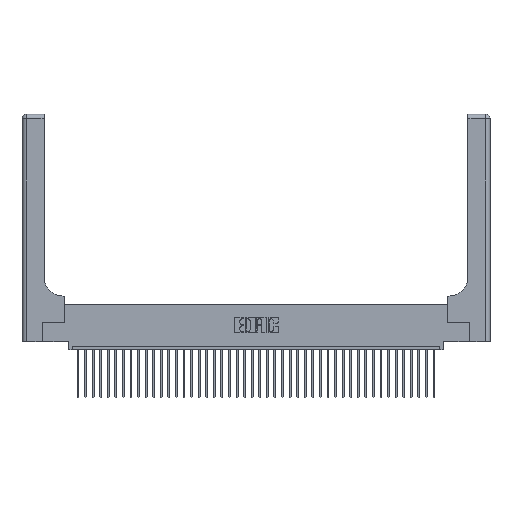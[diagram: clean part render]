
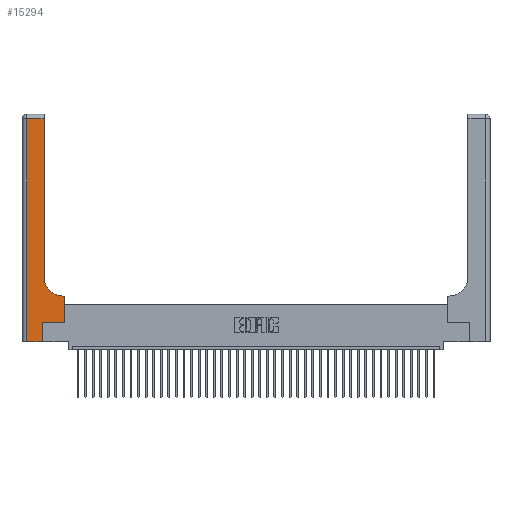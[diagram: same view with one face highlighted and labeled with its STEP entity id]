
A CAD part, top view. The second image highlights one B-rep face of the part: STEP entity #15294.
In plain terms, the highlighted planar face has unit normal (0, 0, 1).
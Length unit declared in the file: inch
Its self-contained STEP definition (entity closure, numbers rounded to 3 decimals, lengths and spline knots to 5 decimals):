
#900 = ORIENTED_EDGE ( 'NONE', *, *, #3843, .T. ) ;
#986 = DIRECTION ( 'NONE',  ( -1., 0., 0. ) ) ;
#2091 = CARTESIAN_POINT ( 'NONE',  ( 0.5585, 0.6, 0.37 ) ) ;
#2290 = EDGE_CURVE ( 'NONE', #22483, #12610, #5214, .T. ) ;
#2780 = CARTESIAN_POINT ( 'NONE',  ( 0.269, 0.25, 0.37 ) ) ;
#3843 = EDGE_CURVE ( 'NONE', #22771, #7628, #37944, .T. ) ;
#5178 = DIRECTION ( 'NONE',  ( -1., 0., 0. ) ) ;
#5214 = LINE ( 'NONE', #17101, #18475 ) ;
#5258 = CARTESIAN_POINT ( 'NONE',  ( 0.269, 0.25, 0.37 ) ) ;
#5501 = EDGE_LOOP ( 'NONE', ( #25806, #17558, #32734, #6866, #40035, #900, #31262, #36947, #14991 ) ) ;
#5596 = CARTESIAN_POINT ( 'NONE',  ( 0., 2.94, 0.37 ) ) ;
#6155 = LINE ( 'NONE', #29979, #15016 ) ;
#6256 = LINE ( 'NONE', #28167, #23412 ) ;
#6866 = ORIENTED_EDGE ( 'NONE', *, *, #17653, .T. ) ;
#6906 = CARTESIAN_POINT ( 'NONE',  ( 0., 0., 0.37 ) ) ;
#7091 = DIRECTION ( 'NONE',  ( 0., 1., 0. ) ) ;
#7136 = VECTOR ( 'NONE', #7091, 39.37008 ) ;
#7628 = VERTEX_POINT ( 'NONE', #33906 ) ;
#9333 = DIRECTION ( 'NONE',  ( 0., 1., 0. ) ) ;
#9922 = DIRECTION ( 'NONE',  ( 0., 0., -1. ) ) ;
#10005 = EDGE_CURVE ( 'NONE', #7628, #14918, #26320, .T. ) ;
#10062 = DIRECTION ( 'NONE',  ( 1., 0., 0. ) ) ;
#10925 = LINE ( 'NONE', #5596, #37979 ) ;
#12610 = VERTEX_POINT ( 'NONE', #15053 ) ;
#14918 = VERTEX_POINT ( 'NONE', #2091 ) ;
#14991 = ORIENTED_EDGE ( 'NONE', *, *, #17389, .T. ) ;
#15016 = VECTOR ( 'NONE', #36300, 39.37008 ) ;
#15053 = CARTESIAN_POINT ( 'NONE',  ( 0.06, 0., 0.37 ) ) ;
#15294 = ADVANCED_FACE ( 'NONE', ( #18983 ), #22891, .F. ) ;
#16080 = AXIS2_PLACEMENT_3D ( 'NONE', #16600, #31807, #986 ) ;
#16600 = CARTESIAN_POINT ( 'NONE',  ( 0., 3., 0.37 ) ) ;
#17101 = CARTESIAN_POINT ( 'NONE',  ( 0.06, 3., 0.37 ) ) ;
#17389 = EDGE_CURVE ( 'NONE', #38373, #29053, #20762, .T. ) ;
#17558 = ORIENTED_EDGE ( 'NONE', *, *, #27865, .T. ) ;
#17653 = EDGE_CURVE ( 'NONE', #12610, #33872, #31529, .T. ) ;
#18475 = VECTOR ( 'NONE', #26286, 39.37008 ) ;
#18750 = CARTESIAN_POINT ( 'NONE',  ( 0.5415, 0.6, 0.37 ) ) ;
#18983 = FACE_OUTER_BOUND ( 'NONE', #5501, .T. ) ;
#19281 = CARTESIAN_POINT ( 'NONE',  ( 0.2915, 0.85, 0.37 ) ) ;
#20571 = EDGE_CURVE ( 'NONE', #29053, #24889, #6256, .T. ) ;
#20762 = CIRCLE ( 'NONE', #39032, 0.25 ) ;
#22190 = VECTOR ( 'NONE', #10062, 39.37008 ) ;
#22483 = VERTEX_POINT ( 'NONE', #37376 ) ;
#22771 = VERTEX_POINT ( 'NONE', #2780 ) ;
#22891 = PLANE ( 'NONE',  #16080 ) ;
#23412 = VECTOR ( 'NONE', #9333, 39.37008 ) ;
#24045 = DIRECTION ( 'NONE',  ( 1., 0., 0. ) ) ;
#24889 = VERTEX_POINT ( 'NONE', #37638 ) ;
#25055 = CARTESIAN_POINT ( 'NONE',  ( 0.5415, 0.85, 0.37 ) ) ;
#25793 = VECTOR ( 'NONE', #33531, 39.37008 ) ;
#25806 = ORIENTED_EDGE ( 'NONE', *, *, #20571, .T. ) ;
#26286 = DIRECTION ( 'NONE',  ( 0., -1., 0. ) ) ;
#26320 = LINE ( 'NONE', #36143, #7136 ) ;
#26797 = EDGE_CURVE ( 'NONE', #33872, #22771, #37182, .T. ) ;
#27865 = EDGE_CURVE ( 'NONE', #24889, #22483, #10925, .T. ) ;
#28167 = CARTESIAN_POINT ( 'NONE',  ( 0.2915, 3., 0.37 ) ) ;
#28488 = DIRECTION ( 'NONE',  ( 1., 0., 0. ) ) ;
#29053 = VERTEX_POINT ( 'NONE', #19281 ) ;
#29979 = CARTESIAN_POINT ( 'NONE',  ( 0.2915, 0.6, 0.37 ) ) ;
#31262 = ORIENTED_EDGE ( 'NONE', *, *, #10005, .T. ) ;
#31529 = LINE ( 'NONE', #6906, #22190 ) ;
#31807 = DIRECTION ( 'NONE',  ( 0., 0., -1. ) ) ;
#32734 = ORIENTED_EDGE ( 'NONE', *, *, #2290, .T. ) ;
#33531 = DIRECTION ( 'NONE',  ( 0., 1., 0. ) ) ;
#33872 = VERTEX_POINT ( 'NONE', #36173 ) ;
#33906 = CARTESIAN_POINT ( 'NONE',  ( 0.5585, 0.25, 0.37 ) ) ;
#35869 = EDGE_CURVE ( 'NONE', #14918, #38373, #6155, .T. ) ;
#36143 = CARTESIAN_POINT ( 'NONE',  ( 0.5585, 0.25, 0.37 ) ) ;
#36173 = CARTESIAN_POINT ( 'NONE',  ( 0.269, 0., 0.37 ) ) ;
#36300 = DIRECTION ( 'NONE',  ( -1., 0., 0. ) ) ;
#36947 = ORIENTED_EDGE ( 'NONE', *, *, #35869, .T. ) ;
#37182 = LINE ( 'NONE', #39549, #25793 ) ;
#37376 = CARTESIAN_POINT ( 'NONE',  ( 0.06, 2.94, 0.37 ) ) ;
#37638 = CARTESIAN_POINT ( 'NONE',  ( 0.2915, 2.94, 0.37 ) ) ;
#37944 = LINE ( 'NONE', #5258, #39920 ) ;
#37979 = VECTOR ( 'NONE', #5178, 39.37008 ) ;
#38373 = VERTEX_POINT ( 'NONE', #18750 ) ;
#39032 = AXIS2_PLACEMENT_3D ( 'NONE', #25055, #9922, #28488 ) ;
#39549 = CARTESIAN_POINT ( 'NONE',  ( 0.269, 0., 0.37 ) ) ;
#39920 = VECTOR ( 'NONE', #24045, 39.37008 ) ;
#40035 = ORIENTED_EDGE ( 'NONE', *, *, #26797, .T. ) ;
